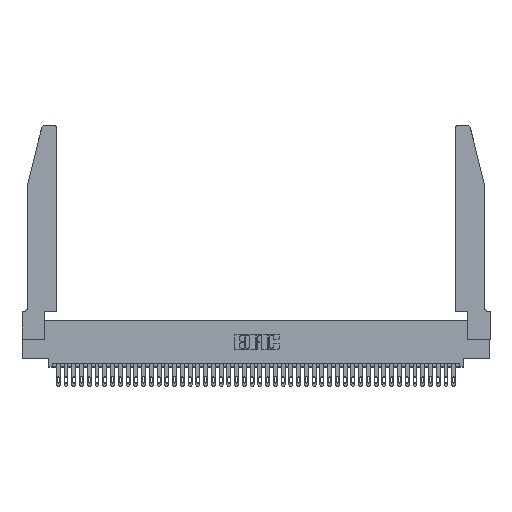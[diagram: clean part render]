
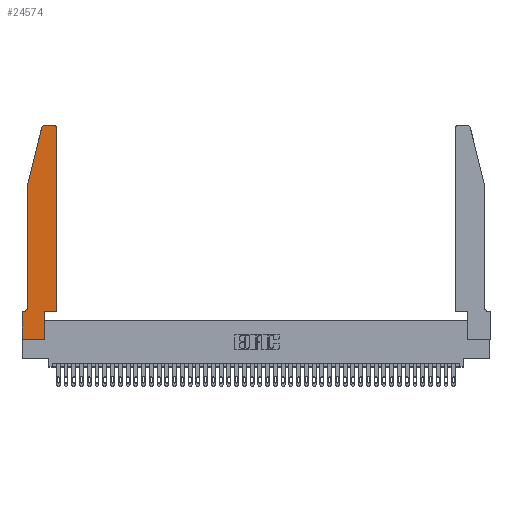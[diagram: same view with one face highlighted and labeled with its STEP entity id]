
A CAD part, top view. The second image highlights one B-rep face of the part: STEP entity #24574.
In plain terms, the highlighted planar face has unit normal (0, 0, 1).
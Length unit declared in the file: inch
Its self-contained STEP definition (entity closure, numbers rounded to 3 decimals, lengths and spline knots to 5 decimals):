
#508 = ORIENTED_EDGE ( 'NONE', *, *, #19030, .T. ) ;
#1476 = ORIENTED_EDGE ( 'NONE', *, *, #10778, .T. ) ;
#1665 = ORIENTED_EDGE ( 'NONE', *, *, #16601, .T. ) ;
#1703 = DIRECTION ( 'NONE',  ( 0., -1., 0. ) ) ;
#2274 = VECTOR ( 'NONE', #41231, 39.37008 ) ;
#2522 = CARTESIAN_POINT ( 'NONE',  ( 0.4505, 2.72, 0.37 ) ) ;
#3551 = DIRECTION ( 'NONE',  ( 1., 0., 0. ) ) ;
#3570 = DIRECTION ( 'NONE',  ( 0., 0., 1. ) ) ;
#3840 = VERTEX_POINT ( 'NONE', #28012 ) ;
#4349 = LINE ( 'NONE', #37470, #35984 ) ;
#4562 = CARTESIAN_POINT ( 'NONE',  ( 0.0755, 0.35, 0.37 ) ) ;
#5084 = EDGE_CURVE ( 'NONE', #29278, #14302, #33556, .T. ) ;
#5836 = ORIENTED_EDGE ( 'NONE', *, *, #11748, .T. ) ;
#6055 = LINE ( 'NONE', #29201, #41358 ) ;
#6719 = PLANE ( 'NONE',  #39523 ) ;
#6901 = ORIENTED_EDGE ( 'NONE', *, *, #5084, .T. ) ;
#7645 = CIRCLE ( 'NONE', #14332, 0.03 ) ;
#7815 = DIRECTION ( 'NONE',  ( -1., 0., 0. ) ) ;
#8051 = CARTESIAN_POINT ( 'NONE',  ( 0.284, 2.72, 0.37 ) ) ;
#8151 = DIRECTION ( 'NONE',  ( -1., 0., 0. ) ) ;
#8668 = LINE ( 'NONE', #30455, #25805 ) ;
#8830 = CARTESIAN_POINT ( 'NONE',  ( 0.2865, 0.35, 0.37 ) ) ;
#8855 = EDGE_CURVE ( 'NONE', #19284, #24820, #35696, .T. ) ;
#8861 = DIRECTION ( 'NONE',  ( 0., 1., 0. ) ) ;
#8948 = EDGE_CURVE ( 'NONE', #24820, #26120, #22305, .T. ) ;
#9884 = CARTESIAN_POINT ( 'NONE',  ( 0.0755, 2., 0.37 ) ) ;
#10409 = CARTESIAN_POINT ( 'NONE',  ( 0.0755, 2., 0.37 ) ) ;
#10624 = ORIENTED_EDGE ( 'NONE', *, *, #21339, .T. ) ;
#10778 = EDGE_CURVE ( 'NONE', #38893, #12172, #7645, .T. ) ;
#10919 = VERTEX_POINT ( 'NONE', #37742 ) ;
#11748 = EDGE_CURVE ( 'NONE', #25655, #10919, #41285, .T. ) ;
#11862 = FACE_OUTER_BOUND ( 'NONE', #15135, .T. ) ;
#12172 = VERTEX_POINT ( 'NONE', #18981 ) ;
#13203 = VECTOR ( 'NONE', #8861, 39.37008 ) ;
#13518 = CARTESIAN_POINT ( 'NONE',  ( 0.4505, 0.35, 0.37 ) ) ;
#13621 = LINE ( 'NONE', #38498, #35034 ) ;
#14116 = DIRECTION ( 'NONE',  ( -1., 0., 0. ) ) ;
#14216 = ORIENTED_EDGE ( 'NONE', *, *, #35256, .T. ) ;
#14302 = VERTEX_POINT ( 'NONE', #31499 ) ;
#14332 = AXIS2_PLACEMENT_3D ( 'NONE', #19594, #27069, #30202 ) ;
#14415 = VECTOR ( 'NONE', #8151, 39.37008 ) ;
#14624 = EDGE_CURVE ( 'NONE', #26120, #15048, #8668, .T. ) ;
#15048 = VERTEX_POINT ( 'NONE', #13518 ) ;
#15135 = EDGE_LOOP ( 'NONE', ( #39525, #6901, #14216, #5836, #10624, #1665, #19968, #39127, #38068, #32144, #508, #1476 ) ) ;
#15957 = AXIS2_PLACEMENT_3D ( 'NONE', #25334, #18463, #7815 ) ;
#16601 = EDGE_CURVE ( 'NONE', #3840, #36485, #25671, .T. ) ;
#18463 = DIRECTION ( 'NONE',  ( 0., 0., -1. ) ) ;
#18526 = CARTESIAN_POINT ( 'NONE',  ( 0., 0.35, 0.37 ) ) ;
#18838 = AXIS2_PLACEMENT_3D ( 'NONE', #8051, #35451, #32294 ) ;
#18981 = CARTESIAN_POINT ( 'NONE',  ( 0.4205, 2.75, 0.37 ) ) ;
#19030 = EDGE_CURVE ( 'NONE', #15048, #38893, #13621, .T. ) ;
#19205 = CARTESIAN_POINT ( 'NONE',  ( 0.2865, 0.35, 0.37 ) ) ;
#19284 = VERTEX_POINT ( 'NONE', #40878 ) ;
#19594 = CARTESIAN_POINT ( 'NONE',  ( 0.4205, 2.72, 0.37 ) ) ;
#19968 = ORIENTED_EDGE ( 'NONE', *, *, #31408, .T. ) ;
#20335 = DIRECTION ( 'NONE',  ( 1., 0., 0. ) ) ;
#21339 = EDGE_CURVE ( 'NONE', #10919, #3840, #43186, .T. ) ;
#22305 = LINE ( 'NONE', #19205, #13203 ) ;
#24416 = VECTOR ( 'NONE', #35655, 39.37008 ) ;
#24574 = ADVANCED_FACE ( 'NONE', ( #11862 ), #6719, .T. ) ;
#24820 = VERTEX_POINT ( 'NONE', #29127 ) ;
#25334 = CARTESIAN_POINT ( 'NONE',  ( 0.0055, 0.42, 0.37 ) ) ;
#25655 = VERTEX_POINT ( 'NONE', #30249 ) ;
#25671 = LINE ( 'NONE', #4562, #14415 ) ;
#25805 = VECTOR ( 'NONE', #3551, 39.37008 ) ;
#26120 = VERTEX_POINT ( 'NONE', #8830 ) ;
#27069 = DIRECTION ( 'NONE',  ( 0., 0., 1. ) ) ;
#28012 = CARTESIAN_POINT ( 'NONE',  ( 0.0055, 0.35, 0.37 ) ) ;
#28293 = VECTOR ( 'NONE', #34358, 39.37008 ) ;
#29127 = CARTESIAN_POINT ( 'NONE',  ( 0.2865, 0., 0.37 ) ) ;
#29201 = CARTESIAN_POINT ( 'NONE',  ( 0., 0., 0.37 ) ) ;
#29278 = VERTEX_POINT ( 'NONE', #31582 ) ;
#30202 = DIRECTION ( 'NONE',  ( 1., 0., 0. ) ) ;
#30249 = CARTESIAN_POINT ( 'NONE',  ( 0.0755, 2., 0.37 ) ) ;
#30455 = CARTESIAN_POINT ( 'NONE',  ( 0.4505, 0.35, 0.37 ) ) ;
#31408 = EDGE_CURVE ( 'NONE', #36485, #19284, #6055, .T. ) ;
#31499 = CARTESIAN_POINT ( 'NONE',  ( 0.25487, 2.72718, 0.37 ) ) ;
#31582 = CARTESIAN_POINT ( 'NONE',  ( 0.284, 2.75, 0.37 ) ) ;
#32144 = ORIENTED_EDGE ( 'NONE', *, *, #14624, .T. ) ;
#32294 = DIRECTION ( 'NONE',  ( 1., 0., 0. ) ) ;
#33556 = CIRCLE ( 'NONE', #18838, 0.03 ) ;
#33886 = EDGE_CURVE ( 'NONE', #12172, #29278, #4349, .T. ) ;
#34358 = DIRECTION ( 'NONE',  ( -0.239, -0.971, 0. ) ) ;
#35034 = VECTOR ( 'NONE', #38642, 39.37008 ) ;
#35256 = EDGE_CURVE ( 'NONE', #14302, #25655, #40611, .T. ) ;
#35451 = DIRECTION ( 'NONE',  ( 0., 0., 1. ) ) ;
#35655 = DIRECTION ( 'NONE',  ( 1., 0., 0. ) ) ;
#35696 = LINE ( 'NONE', #41320, #24416 ) ;
#35984 = VECTOR ( 'NONE', #14116, 39.37008 ) ;
#36485 = VERTEX_POINT ( 'NONE', #18526 ) ;
#37470 = CARTESIAN_POINT ( 'NONE',  ( 0.2605, 2.75, 0.37 ) ) ;
#37742 = CARTESIAN_POINT ( 'NONE',  ( 0.0755, 0.42, 0.37 ) ) ;
#38068 = ORIENTED_EDGE ( 'NONE', *, *, #8948, .T. ) ;
#38498 = CARTESIAN_POINT ( 'NONE',  ( 0.4505, 0.35, 0.37 ) ) ;
#38642 = DIRECTION ( 'NONE',  ( 0., 1., 0. ) ) ;
#38893 = VERTEX_POINT ( 'NONE', #2522 ) ;
#39127 = ORIENTED_EDGE ( 'NONE', *, *, #8855, .T. ) ;
#39523 = AXIS2_PLACEMENT_3D ( 'NONE', #40794, #3570, #20335 ) ;
#39525 = ORIENTED_EDGE ( 'NONE', *, *, #33886, .T. ) ;
#40611 = LINE ( 'NONE', #10409, #28293 ) ;
#40794 = CARTESIAN_POINT ( 'NONE',  ( 0., 0.35, 0.37 ) ) ;
#40878 = CARTESIAN_POINT ( 'NONE',  ( 0., 0., 0.37 ) ) ;
#41231 = DIRECTION ( 'NONE',  ( 0., -1., 0. ) ) ;
#41285 = LINE ( 'NONE', #9884, #2274 ) ;
#41320 = CARTESIAN_POINT ( 'NONE',  ( 0., 0., 0.37 ) ) ;
#41358 = VECTOR ( 'NONE', #1703, 39.37008 ) ;
#43186 = CIRCLE ( 'NONE', #15957, 0.07 ) ;
